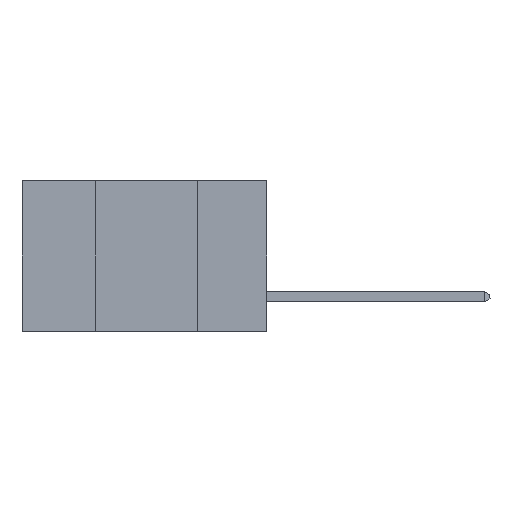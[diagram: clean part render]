
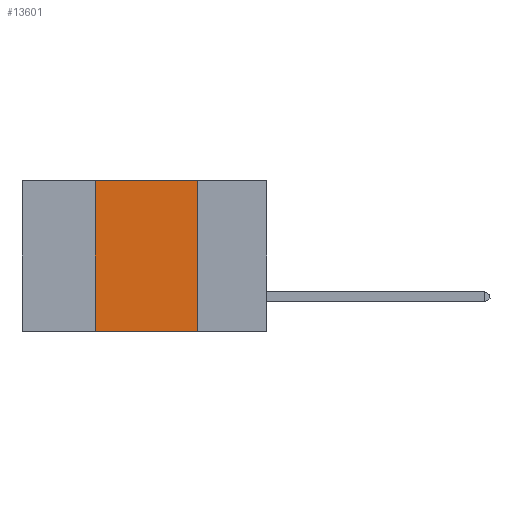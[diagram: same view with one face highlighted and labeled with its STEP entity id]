
A CAD part, left-side view. The second image highlights one B-rep face of the part: STEP entity #13601.
In plain terms, the highlighted planar face has unit normal (-1, 0, 0).
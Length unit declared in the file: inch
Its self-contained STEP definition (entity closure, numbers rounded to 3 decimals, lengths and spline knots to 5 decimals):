
#295 = LINE ( 'NONE', #7696, #5070 ) ;
#1016 = DIRECTION ( 'NONE',  ( 0., -1., 0. ) ) ;
#1467 = ORIENTED_EDGE ( 'NONE', *, *, #14325, .T. ) ;
#2852 = VERTEX_POINT ( 'NONE', #5766 ) ;
#2907 = FACE_OUTER_BOUND ( 'NONE', #15721, .T. ) ;
#3427 = VERTEX_POINT ( 'NONE', #8718 ) ;
#3925 = LINE ( 'NONE', #4000, #19205 ) ;
#4000 = CARTESIAN_POINT ( 'NONE',  ( 0., 0.42, 0. ) ) ;
#5070 = VECTOR ( 'NONE', #7627, 39.37008 ) ;
#5766 = CARTESIAN_POINT ( 'NONE',  ( 0., 0.17, 0. ) ) ;
#7104 = DIRECTION ( 'NONE',  ( 0., 0., 1. ) ) ;
#7147 = PLANE ( 'NONE',  #19951 ) ;
#7627 = DIRECTION ( 'NONE',  ( 0., 0., -1. ) ) ;
#7696 = CARTESIAN_POINT ( 'NONE',  ( 0., 0.17, 0. ) ) ;
#8688 = DIRECTION ( 'NONE',  ( 0., 0., -1. ) ) ;
#8718 = CARTESIAN_POINT ( 'NONE',  ( 0., 0.42, 0. ) ) ;
#9412 = DIRECTION ( 'NONE',  ( 0., -1., 0. ) ) ;
#9974 = VERTEX_POINT ( 'NONE', #16156 ) ;
#10113 = ORIENTED_EDGE ( 'NONE', *, *, #15370, .F. ) ;
#11633 = ORIENTED_EDGE ( 'NONE', *, *, #17681, .F. ) ;
#11889 = VECTOR ( 'NONE', #9412, 39.37008 ) ;
#12115 = ORIENTED_EDGE ( 'NONE', *, *, #14526, .F. ) ;
#12132 = VERTEX_POINT ( 'NONE', #12755 ) ;
#12755 = CARTESIAN_POINT ( 'NONE',  ( 0., 0.17, -0.37 ) ) ;
#13305 = CARTESIAN_POINT ( 'NONE',  ( 0., 0.6, 0. ) ) ;
#13601 = ADVANCED_FACE ( 'NONE', ( #2907 ), #7147, .F. ) ;
#13613 = LINE ( 'NONE', #16513, #16140 ) ;
#14325 = EDGE_CURVE ( 'NONE', #9974, #12132, #13613, .T. ) ;
#14526 = EDGE_CURVE ( 'NONE', #3427, #2852, #16831, .T. ) ;
#15370 = EDGE_CURVE ( 'NONE', #2852, #12132, #295, .T. ) ;
#15721 = EDGE_LOOP ( 'NONE', ( #10113, #12115, #11633, #1467 ) ) ;
#16140 = VECTOR ( 'NONE', #1016, 39.37008 ) ;
#16156 = CARTESIAN_POINT ( 'NONE',  ( 0., 0.42, -0.37 ) ) ;
#16513 = CARTESIAN_POINT ( 'NONE',  ( 0., 0.6, -0.37 ) ) ;
#16831 = LINE ( 'NONE', #19946, #11889 ) ;
#17681 = EDGE_CURVE ( 'NONE', #9974, #3427, #3925, .T. ) ;
#17769 = DIRECTION ( 'NONE',  ( 1., 0., 0. ) ) ;
#19205 = VECTOR ( 'NONE', #7104, 39.37008 ) ;
#19946 = CARTESIAN_POINT ( 'NONE',  ( 0., 0.6, 0. ) ) ;
#19951 = AXIS2_PLACEMENT_3D ( 'NONE', #13305, #17769, #8688 ) ;
